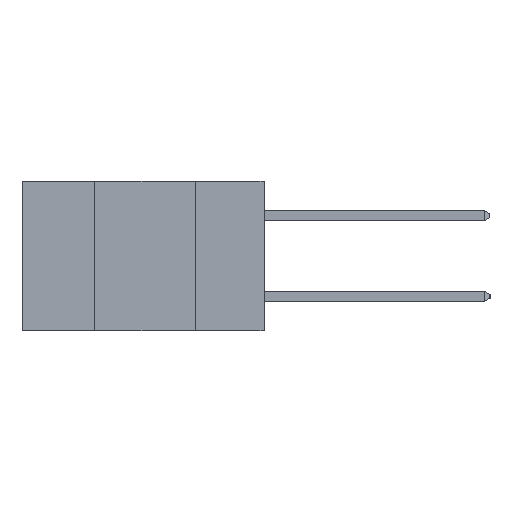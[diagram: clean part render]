
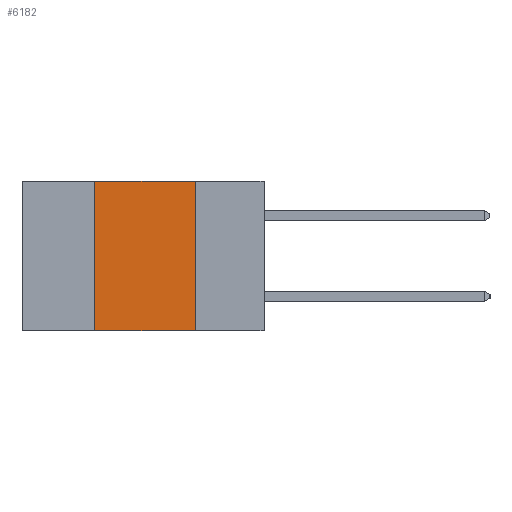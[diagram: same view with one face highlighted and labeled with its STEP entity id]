
A CAD part, left-side view. The second image highlights one B-rep face of the part: STEP entity #6182.
In plain terms, the highlighted planar face has unit normal (-1, 0, 0).
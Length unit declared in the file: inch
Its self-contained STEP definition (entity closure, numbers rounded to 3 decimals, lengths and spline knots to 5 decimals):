
#106 = VECTOR ( 'NONE', #8436, 39.37008 ) ;
#461 = CARTESIAN_POINT ( 'NONE',  ( 0., 0.17, -0.37 ) ) ;
#1106 = VERTEX_POINT ( 'NONE', #17259 ) ;
#1151 = VECTOR ( 'NONE', #2896, 39.37008 ) ;
#1574 = ORIENTED_EDGE ( 'NONE', *, *, #17150, .F. ) ;
#2648 = DIRECTION ( 'NONE',  ( 0., -1., 0. ) ) ;
#2763 = CARTESIAN_POINT ( 'NONE',  ( 0., 0.6, -0.37 ) ) ;
#2896 = DIRECTION ( 'NONE',  ( 0., 0., 1. ) ) ;
#3120 = CARTESIAN_POINT ( 'NONE',  ( 0., 0.42, -0.37 ) ) ;
#4680 = VERTEX_POINT ( 'NONE', #9354 ) ;
#5372 = LINE ( 'NONE', #3120, #1151 ) ;
#5408 = EDGE_CURVE ( 'NONE', #11872, #1106, #5372, .T. ) ;
#6182 = ADVANCED_FACE ( 'NONE', ( #15789 ), #11363, .F. ) ;
#6414 = ORIENTED_EDGE ( 'NONE', *, *, #7140, .T. ) ;
#6734 = LINE ( 'NONE', #17583, #15897 ) ;
#7140 = EDGE_CURVE ( 'NONE', #11872, #18158, #16668, .T. ) ;
#7498 = EDGE_LOOP ( 'NONE', ( #14092, #1574, #11219, #6414 ) ) ;
#8436 = DIRECTION ( 'NONE',  ( 0., 0., -1. ) ) ;
#8448 = DIRECTION ( 'NONE',  ( 0., -1., 0. ) ) ;
#9017 = AXIS2_PLACEMENT_3D ( 'NONE', #11850, #11162, #11074 ) ;
#9354 = CARTESIAN_POINT ( 'NONE',  ( 0., 0.17, 0. ) ) ;
#11074 = DIRECTION ( 'NONE',  ( 0., 0., -1. ) ) ;
#11162 = DIRECTION ( 'NONE',  ( 1., 0., 0. ) ) ;
#11219 = ORIENTED_EDGE ( 'NONE', *, *, #5408, .F. ) ;
#11363 = PLANE ( 'NONE',  #9017 ) ;
#11850 = CARTESIAN_POINT ( 'NONE',  ( 0., 0.6, 0. ) ) ;
#11872 = VERTEX_POINT ( 'NONE', #18365 ) ;
#12222 = VECTOR ( 'NONE', #2648, 39.37008 ) ;
#12696 = LINE ( 'NONE', #461, #106 ) ;
#14092 = ORIENTED_EDGE ( 'NONE', *, *, #15167, .F. ) ;
#15167 = EDGE_CURVE ( 'NONE', #4680, #18158, #12696, .T. ) ;
#15789 = FACE_OUTER_BOUND ( 'NONE', #7498, .T. ) ;
#15897 = VECTOR ( 'NONE', #8448, 39.37008 ) ;
#16668 = LINE ( 'NONE', #2763, #12222 ) ;
#16814 = CARTESIAN_POINT ( 'NONE',  ( 0., 0.17, -0.37 ) ) ;
#17150 = EDGE_CURVE ( 'NONE', #1106, #4680, #6734, .T. ) ;
#17259 = CARTESIAN_POINT ( 'NONE',  ( 0., 0.42, 0. ) ) ;
#17583 = CARTESIAN_POINT ( 'NONE',  ( 0., 0.6, 0. ) ) ;
#18158 = VERTEX_POINT ( 'NONE', #16814 ) ;
#18365 = CARTESIAN_POINT ( 'NONE',  ( 0., 0.42, -0.37 ) ) ;
